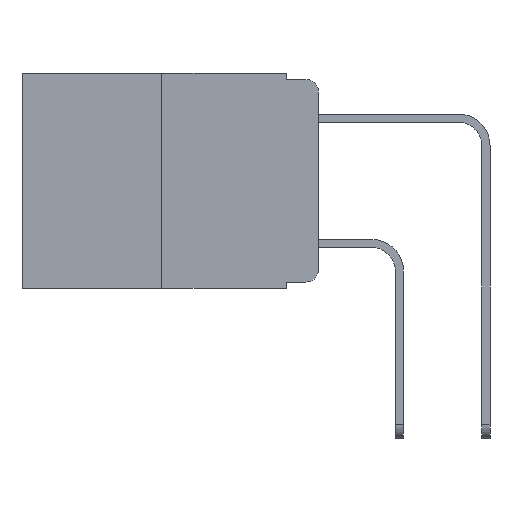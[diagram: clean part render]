
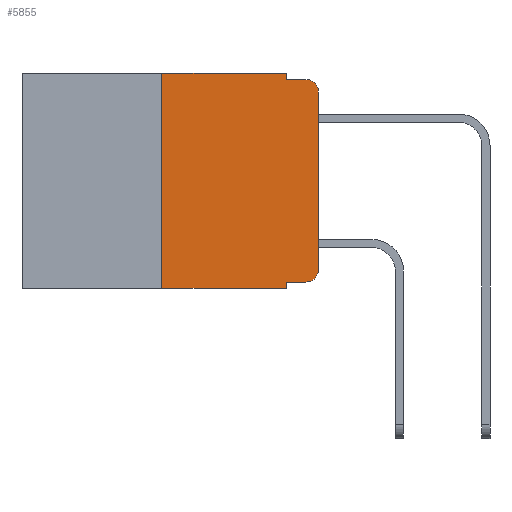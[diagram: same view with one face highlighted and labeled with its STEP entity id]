
A CAD part, left-side view. The second image highlights one B-rep face of the part: STEP entity #5855.
In plain terms, the highlighted planar face has unit normal (-1, 0, 0).
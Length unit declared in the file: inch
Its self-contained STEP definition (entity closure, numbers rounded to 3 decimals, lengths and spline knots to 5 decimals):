
#315 = VECTOR ( 'NONE', #3589, 39.37008 ) ;
#731 = ORIENTED_EDGE ( 'NONE', *, *, #8178, .F. ) ;
#990 = VERTEX_POINT ( 'NONE', #11997 ) ;
#1016 = DIRECTION ( 'NONE',  ( 0., -1., 0. ) ) ;
#1038 = VERTEX_POINT ( 'NONE', #2389 ) ;
#1073 = ORIENTED_EDGE ( 'NONE', *, *, #1225, .T. ) ;
#1085 = CARTESIAN_POINT ( 'NONE',  ( 0., 0.02, -0.313 ) ) ;
#1171 = DIRECTION ( 'NONE',  ( -1., 0., 0. ) ) ;
#1225 = EDGE_CURVE ( 'NONE', #5893, #2263, #3607, .T. ) ;
#1418 = VERTEX_POINT ( 'NONE', #6989 ) ;
#1699 = VERTEX_POINT ( 'NONE', #4361 ) ;
#1829 = EDGE_CURVE ( 'NONE', #1038, #3379, #4964, .T. ) ;
#2263 = VERTEX_POINT ( 'NONE', #2395 ) ;
#2278 = VECTOR ( 'NONE', #5922, 39.37008 ) ;
#2316 = CARTESIAN_POINT ( 'NONE',  ( 0., 0.051, 0. ) ) ;
#2328 = LINE ( 'NONE', #5571, #12430 ) ;
#2371 = VECTOR ( 'NONE', #3137, 39.37008 ) ;
#2389 = CARTESIAN_POINT ( 'NONE',  ( 0., 0.25, 0. ) ) ;
#2395 = CARTESIAN_POINT ( 'NONE',  ( 0., 0.02, -0.01 ) ) ;
#2489 = VERTEX_POINT ( 'NONE', #7591 ) ;
#2560 = DIRECTION ( 'NONE',  ( 0., 0., 1. ) ) ;
#2672 = VECTOR ( 'NONE', #1016, 39.37008 ) ;
#2689 = LINE ( 'NONE', #11151, #3819 ) ;
#2720 = ORIENTED_EDGE ( 'NONE', *, *, #12054, .T. ) ;
#2894 = EDGE_CURVE ( 'NONE', #1418, #990, #3712, .T. ) ;
#2947 = DIRECTION ( 'NONE',  ( -1., 0., 0. ) ) ;
#3005 = LINE ( 'NONE', #9313, #2672 ) ;
#3079 = DIRECTION ( 'NONE',  ( 0., 0., -1. ) ) ;
#3136 = LINE ( 'NONE', #7995, #315 ) ;
#3137 = DIRECTION ( 'NONE',  ( 0., 0., -1. ) ) ;
#3379 = VERTEX_POINT ( 'NONE', #2316 ) ;
#3417 = VERTEX_POINT ( 'NONE', #12820 ) ;
#3589 = DIRECTION ( 'NONE',  ( 0., -1., 0. ) ) ;
#3594 = EDGE_CURVE ( 'NONE', #990, #1699, #6472, .T. ) ;
#3607 = CIRCLE ( 'NONE', #10726, 0.02 ) ;
#3712 = LINE ( 'NONE', #5151, #8012 ) ;
#3819 = VECTOR ( 'NONE', #8270, 39.37008 ) ;
#4162 = CARTESIAN_POINT ( 'NONE',  ( 0., 0.473, 0. ) ) ;
#4361 = CARTESIAN_POINT ( 'NONE',  ( 0., 0., -0.313 ) ) ;
#4379 = PLANE ( 'NONE',  #10283 ) ;
#4641 = ORIENTED_EDGE ( 'NONE', *, *, #1829, .F. ) ;
#4905 = EDGE_CURVE ( 'NONE', #2489, #1038, #5522, .T. ) ;
#4964 = LINE ( 'NONE', #5069, #2278 ) ;
#5069 = CARTESIAN_POINT ( 'NONE',  ( 0., 0.473, 0. ) ) ;
#5081 = EDGE_CURVE ( 'NONE', #2489, #7152, #3005, .T. ) ;
#5151 = CARTESIAN_POINT ( 'NONE',  ( 0., 0.051, -0.333 ) ) ;
#5522 = LINE ( 'NONE', #12308, #8101 ) ;
#5571 = CARTESIAN_POINT ( 'NONE',  ( 0., 0., 0. ) ) ;
#5855 = ADVANCED_FACE ( 'NONE', ( #6846 ), #4379, .F. ) ;
#5890 = DIRECTION ( 'NONE',  ( 0., 0., -1. ) ) ;
#5893 = VERTEX_POINT ( 'NONE', #10803 ) ;
#5922 = DIRECTION ( 'NONE',  ( 0., -1., 0. ) ) ;
#6472 = CIRCLE ( 'NONE', #11533, 0.02 ) ;
#6777 = CARTESIAN_POINT ( 'NONE',  ( 0., 0.051, -0.343 ) ) ;
#6846 = FACE_OUTER_BOUND ( 'NONE', #10336, .T. ) ;
#6868 = EDGE_CURVE ( 'NONE', #1418, #7152, #2689, .T. ) ;
#6989 = CARTESIAN_POINT ( 'NONE',  ( 0., 0.051, -0.333 ) ) ;
#7152 = VERTEX_POINT ( 'NONE', #6777 ) ;
#7591 = CARTESIAN_POINT ( 'NONE',  ( 0., 0.25, -0.343 ) ) ;
#7995 = CARTESIAN_POINT ( 'NONE',  ( 0., 0.051, -0.01 ) ) ;
#8012 = VECTOR ( 'NONE', #10545, 39.37008 ) ;
#8047 = ORIENTED_EDGE ( 'NONE', *, *, #6868, .F. ) ;
#8101 = VECTOR ( 'NONE', #8288, 39.37008 ) ;
#8177 = DIRECTION ( 'NONE',  ( 0., 0., -1. ) ) ;
#8178 = EDGE_CURVE ( 'NONE', #3417, #2263, #3136, .T. ) ;
#8270 = DIRECTION ( 'NONE',  ( 0., 0., -1. ) ) ;
#8288 = DIRECTION ( 'NONE',  ( 0., 0., 1. ) ) ;
#8938 = ORIENTED_EDGE ( 'NONE', *, *, #2894, .T. ) ;
#9313 = CARTESIAN_POINT ( 'NONE',  ( 0., 0.473, -0.343 ) ) ;
#9699 = ORIENTED_EDGE ( 'NONE', *, *, #5081, .T. ) ;
#9708 = ORIENTED_EDGE ( 'NONE', *, *, #4905, .F. ) ;
#9912 = ORIENTED_EDGE ( 'NONE', *, *, #10777, .F. ) ;
#9992 = CARTESIAN_POINT ( 'NONE',  ( 0., 0.051, 0. ) ) ;
#10239 = LINE ( 'NONE', #9992, #2371 ) ;
#10283 = AXIS2_PLACEMENT_3D ( 'NONE', #4162, #12541, #5890 ) ;
#10336 = EDGE_LOOP ( 'NONE', ( #2720, #1073, #731, #9912, #4641, #9708, #9699, #8047, #8938, #11491 ) ) ;
#10545 = DIRECTION ( 'NONE',  ( 0., -1., 0. ) ) ;
#10726 = AXIS2_PLACEMENT_3D ( 'NONE', #11395, #2947, #3079 ) ;
#10777 = EDGE_CURVE ( 'NONE', #3379, #3417, #10239, .T. ) ;
#10803 = CARTESIAN_POINT ( 'NONE',  ( 0., 0., -0.03 ) ) ;
#11151 = CARTESIAN_POINT ( 'NONE',  ( 0., 0.051, 0. ) ) ;
#11395 = CARTESIAN_POINT ( 'NONE',  ( 0., 0.02, -0.03 ) ) ;
#11491 = ORIENTED_EDGE ( 'NONE', *, *, #3594, .T. ) ;
#11533 = AXIS2_PLACEMENT_3D ( 'NONE', #1085, #1171, #8177 ) ;
#11997 = CARTESIAN_POINT ( 'NONE',  ( 0., 0.02, -0.333 ) ) ;
#12054 = EDGE_CURVE ( 'NONE', #1699, #5893, #2328, .T. ) ;
#12308 = CARTESIAN_POINT ( 'NONE',  ( 0., 0.25, 0. ) ) ;
#12430 = VECTOR ( 'NONE', #2560, 39.37008 ) ;
#12541 = DIRECTION ( 'NONE',  ( 1., 0., 0. ) ) ;
#12820 = CARTESIAN_POINT ( 'NONE',  ( 0., 0.051, -0.01 ) ) ;
